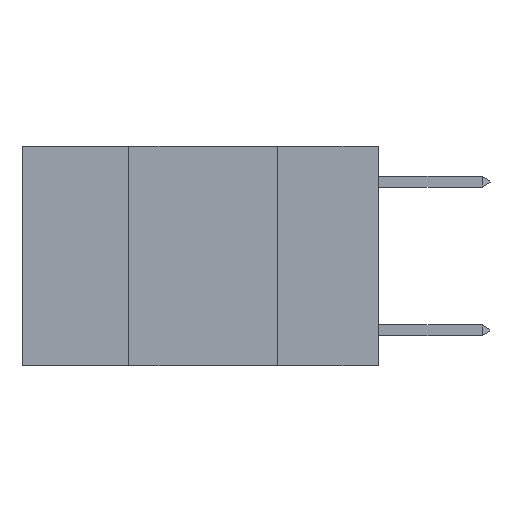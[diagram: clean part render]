
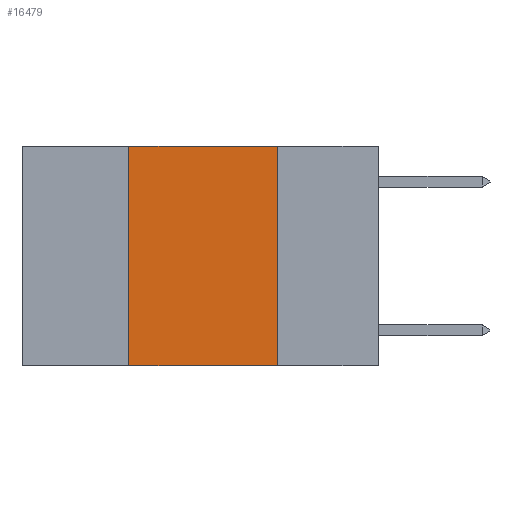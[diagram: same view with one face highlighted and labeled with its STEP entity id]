
A CAD part, left-side view. The second image highlights one B-rep face of the part: STEP entity #16479.
In plain terms, the highlighted planar face has unit normal (-1, 0, 0).
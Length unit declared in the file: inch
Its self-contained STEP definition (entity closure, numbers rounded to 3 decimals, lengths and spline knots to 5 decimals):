
#525 = CARTESIAN_POINT ( 'NONE',  ( 0., 0.6, 0. ) ) ;
#3189 = LINE ( 'NONE', #6708, #27348 ) ;
#4729 = AXIS2_PLACEMENT_3D ( 'NONE', #24384, #29358, #14981 ) ;
#4869 = EDGE_CURVE ( 'NONE', #22766, #11903, #19187, .T. ) ;
#4957 = DIRECTION ( 'NONE',  ( 0., 0., 1. ) ) ;
#4988 = CARTESIAN_POINT ( 'NONE',  ( 0., 0.42, 0. ) ) ;
#5653 = EDGE_LOOP ( 'NONE', ( #16795, #17336, #17859, #17913 ) ) ;
#5670 = VECTOR ( 'NONE', #4957, 39.37008 ) ;
#6708 = CARTESIAN_POINT ( 'NONE',  ( 0., 0.17, 0. ) ) ;
#7342 = FACE_OUTER_BOUND ( 'NONE', #5653, .T. ) ;
#9160 = DIRECTION ( 'NONE',  ( 0., 0., -1. ) ) ;
#10559 = CARTESIAN_POINT ( 'NONE',  ( 0., 0.42, 0. ) ) ;
#10598 = CARTESIAN_POINT ( 'NONE',  ( 0., 0.6, -0.37 ) ) ;
#11255 = EDGE_CURVE ( 'NONE', #22766, #30851, #16056, .T. ) ;
#11903 = VERTEX_POINT ( 'NONE', #10559 ) ;
#14981 = DIRECTION ( 'NONE',  ( 0., 0., -1. ) ) ;
#15300 = VECTOR ( 'NONE', #17791, 39.37008 ) ;
#16056 = LINE ( 'NONE', #10598, #15300 ) ;
#16458 = CARTESIAN_POINT ( 'NONE',  ( 0., 0.42, -0.37 ) ) ;
#16479 = ADVANCED_FACE ( 'NONE', ( #7342 ), #29161, .F. ) ;
#16795 = ORIENTED_EDGE ( 'NONE', *, *, #27000, .F. ) ;
#17336 = ORIENTED_EDGE ( 'NONE', *, *, #30573, .F. ) ;
#17791 = DIRECTION ( 'NONE',  ( 0., -1., 0. ) ) ;
#17859 = ORIENTED_EDGE ( 'NONE', *, *, #4869, .F. ) ;
#17913 = ORIENTED_EDGE ( 'NONE', *, *, #11255, .T. ) ;
#19187 = LINE ( 'NONE', #4988, #5670 ) ;
#22321 = DIRECTION ( 'NONE',  ( 0., -1., 0. ) ) ;
#22766 = VERTEX_POINT ( 'NONE', #16458 ) ;
#22927 = VECTOR ( 'NONE', #22321, 39.37008 ) ;
#23267 = CARTESIAN_POINT ( 'NONE',  ( 0., 0.17, -0.37 ) ) ;
#23439 = VERTEX_POINT ( 'NONE', #23528 ) ;
#23528 = CARTESIAN_POINT ( 'NONE',  ( 0., 0.17, 0. ) ) ;
#24384 = CARTESIAN_POINT ( 'NONE',  ( 0., 0.6, 0. ) ) ;
#27000 = EDGE_CURVE ( 'NONE', #23439, #30851, #3189, .T. ) ;
#27348 = VECTOR ( 'NONE', #9160, 39.37008 ) ;
#29161 = PLANE ( 'NONE',  #4729 ) ;
#29358 = DIRECTION ( 'NONE',  ( 1., 0., 0. ) ) ;
#30573 = EDGE_CURVE ( 'NONE', #11903, #23439, #30897, .T. ) ;
#30851 = VERTEX_POINT ( 'NONE', #23267 ) ;
#30897 = LINE ( 'NONE', #525, #22927 ) ;
